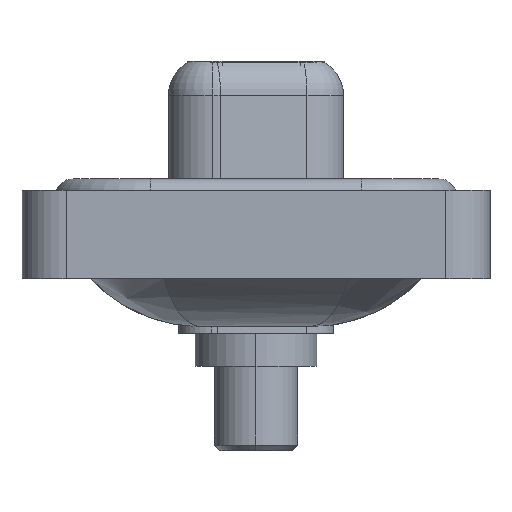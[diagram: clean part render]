
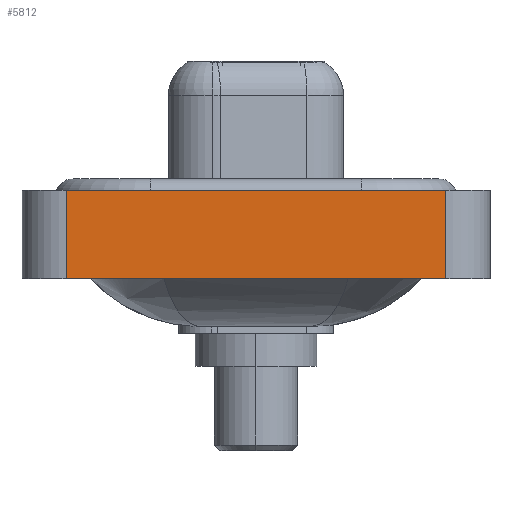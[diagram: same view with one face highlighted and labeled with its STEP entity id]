
A CAD part, left-side view. The second image highlights one B-rep face of the part: STEP entity #5812.
In plain terms, the highlighted planar face has unit normal (-1, 0, 0).
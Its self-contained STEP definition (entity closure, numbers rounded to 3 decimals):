
#403 = LINE ( 'NONE', #15016, #16144 ) ;
#519 = EDGE_CURVE ( 'NONE', #13233, #8397, #8034, .T. ) ;
#704 = EDGE_CURVE ( 'NONE', #13233, #7271, #10117, .T. ) ;
#1122 = AXIS2_PLACEMENT_3D ( 'NONE', #12943, #14108, #4654 ) ;
#1256 = DIRECTION ( 'NONE',  ( 0., 0., 1. ) ) ;
#3311 = PLANE ( 'NONE',  #1122 ) ;
#4269 = EDGE_LOOP ( 'NONE', ( #10891, #15151, #5397, #10581 ) ) ;
#4654 = DIRECTION ( 'NONE',  ( 0., 0., 1. ) ) ;
#4746 = CARTESIAN_POINT ( 'NONE',  ( -7.3, 8.55, -3.6 ) ) ;
#4790 = DIRECTION ( 'NONE',  ( 0., -1., 0. ) ) ;
#5397 = ORIENTED_EDGE ( 'NONE', *, *, #519, .F. ) ;
#5649 = DIRECTION ( 'NONE',  ( 0., 0., 1. ) ) ;
#5763 = CARTESIAN_POINT ( 'NONE',  ( -7.3, -8.55, 0.4 ) ) ;
#5802 = DIRECTION ( 'NONE',  ( 0., -1., 0. ) ) ;
#5812 = ADVANCED_FACE ( 'NONE', ( #12683 ), #3311, .T. ) ;
#6380 = CARTESIAN_POINT ( 'NONE',  ( -7.3, 8.55, 0.4 ) ) ;
#7271 = VERTEX_POINT ( 'NONE', #7877 ) ;
#7418 = VECTOR ( 'NONE', #1256, 1000. ) ;
#7877 = CARTESIAN_POINT ( 'NONE',  ( -7.3, -8.55, -3.6 ) ) ;
#8034 = LINE ( 'NONE', #14817, #7418 ) ;
#8397 = VERTEX_POINT ( 'NONE', #6380 ) ;
#10117 = LINE ( 'NONE', #11519, #13870 ) ;
#10581 = ORIENTED_EDGE ( 'NONE', *, *, #704, .T. ) ;
#10891 = ORIENTED_EDGE ( 'NONE', *, *, #14589, .T. ) ;
#11519 = CARTESIAN_POINT ( 'NONE',  ( -7.3, -8.55, -3.6 ) ) ;
#12683 = FACE_OUTER_BOUND ( 'NONE', #4269, .T. ) ;
#12943 = CARTESIAN_POINT ( 'NONE',  ( -7.3, -8.55, -3.6 ) ) ;
#13233 = VERTEX_POINT ( 'NONE', #4746 ) ;
#13870 = VECTOR ( 'NONE', #4790, 1000. ) ;
#13936 = LINE ( 'NONE', #14899, #15010 ) ;
#14018 = VERTEX_POINT ( 'NONE', #5763 ) ;
#14108 = DIRECTION ( 'NONE',  ( -1., 0., 0. ) ) ;
#14589 = EDGE_CURVE ( 'NONE', #7271, #14018, #403, .T. ) ;
#14817 = CARTESIAN_POINT ( 'NONE',  ( -7.3, 8.55, -3.6 ) ) ;
#14899 = CARTESIAN_POINT ( 'NONE',  ( -7.3, -8.55, 0.4 ) ) ;
#14960 = EDGE_CURVE ( 'NONE', #8397, #14018, #13936, .T. ) ;
#15010 = VECTOR ( 'NONE', #5802, 1000. ) ;
#15016 = CARTESIAN_POINT ( 'NONE',  ( -7.3, -8.55, -3.6 ) ) ;
#15151 = ORIENTED_EDGE ( 'NONE', *, *, #14960, .F. ) ;
#16144 = VECTOR ( 'NONE', #5649, 1000. ) ;
